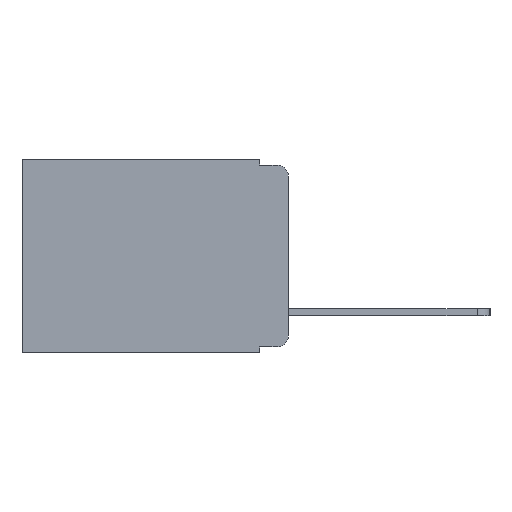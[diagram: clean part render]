
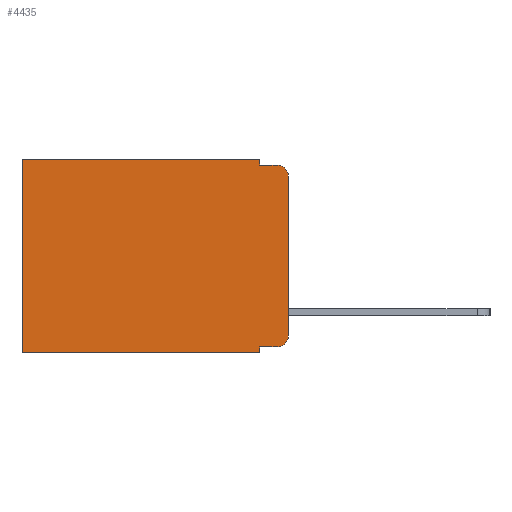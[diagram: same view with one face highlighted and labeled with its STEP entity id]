
A CAD part, left-side view. The second image highlights one B-rep face of the part: STEP entity #4435.
In plain terms, the highlighted planar face has unit normal (-1, 0, 0).
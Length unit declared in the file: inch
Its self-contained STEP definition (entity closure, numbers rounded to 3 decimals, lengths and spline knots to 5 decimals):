
#233 = ORIENTED_EDGE ( 'NONE', *, *, #13296, .F. ) ;
#249 = ORIENTED_EDGE ( 'NONE', *, *, #522, .T. ) ;
#310 = VERTEX_POINT ( 'NONE', #15854 ) ;
#501 = FACE_OUTER_BOUND ( 'NONE', #6008, .T. ) ;
#522 = EDGE_CURVE ( 'NONE', #1548, #3843, #5120, .T. ) ;
#576 = DIRECTION ( 'NONE',  ( 0., 1., 0. ) ) ;
#608 = DIRECTION ( 'NONE',  ( 0., -1., 0. ) ) ;
#623 = CARTESIAN_POINT ( 'NONE',  ( 0.298, 0., 0. ) ) ;
#873 = ORIENTED_EDGE ( 'NONE', *, *, #13072, .T. ) ;
#1028 = ORIENTED_EDGE ( 'NONE', *, *, #13233, .F. ) ;
#1104 = DIRECTION ( 'NONE',  ( 0., 0., -1. ) ) ;
#1265 = CARTESIAN_POINT ( 'NONE',  ( 0.298, 0., 0. ) ) ;
#1548 = VERTEX_POINT ( 'NONE', #4583 ) ;
#1913 = VERTEX_POINT ( 'NONE', #6300 ) ;
#2069 = ORIENTED_EDGE ( 'NONE', *, *, #13324, .T. ) ;
#2408 = VECTOR ( 'NONE', #576, 39.37008 ) ;
#3073 = VERTEX_POINT ( 'NONE', #6090 ) ;
#3367 = ORIENTED_EDGE ( 'NONE', *, *, #11075, .F. ) ;
#3386 = DIRECTION ( 'NONE',  ( 0., 1., 0. ) ) ;
#3620 = VECTOR ( 'NONE', #6808, 39.37008 ) ;
#3739 = CARTESIAN_POINT ( 'NONE',  ( 0.298, 0.051, -0.333 ) ) ;
#3843 = VERTEX_POINT ( 'NONE', #13673 ) ;
#4435 = ADVANCED_FACE ( 'NONE', ( #501 ), #11985, .F. ) ;
#4469 = DIRECTION ( 'NONE',  ( 0., 0., -1. ) ) ;
#4554 = CARTESIAN_POINT ( 'NONE',  ( 0.298, 0.473, -0.343 ) ) ;
#4583 = CARTESIAN_POINT ( 'NONE',  ( 0.298, 0.051, 0. ) ) ;
#4594 = LINE ( 'NONE', #18398, #18764 ) ;
#4664 = DIRECTION ( 'NONE',  ( -1., 0., 0. ) ) ;
#4992 = ORIENTED_EDGE ( 'NONE', *, *, #13290, .T. ) ;
#5120 = LINE ( 'NONE', #623, #2408 ) ;
#5637 = ORIENTED_EDGE ( 'NONE', *, *, #13431, .T. ) ;
#5700 = AXIS2_PLACEMENT_3D ( 'NONE', #18890, #10250, #1104 ) ;
#6008 = EDGE_LOOP ( 'NONE', ( #17667, #873, #18795, #1028, #249, #4992, #3367, #233, #2069, #5637 ) ) ;
#6090 = CARTESIAN_POINT ( 'NONE',  ( 0.298, 0., -0.03 ) ) ;
#6300 = CARTESIAN_POINT ( 'NONE',  ( 0.298, 0.02, -0.01 ) ) ;
#6516 = DIRECTION ( 'NONE',  ( 1., 0., 0. ) ) ;
#6535 = DIRECTION ( 'NONE',  ( 0., 0., -1. ) ) ;
#6622 = CARTESIAN_POINT ( 'NONE',  ( 0.298, 0.051, 0. ) ) ;
#6697 = LINE ( 'NONE', #8375, #14943 ) ;
#6808 = DIRECTION ( 'NONE',  ( 0., 0., -1. ) ) ;
#7389 = CIRCLE ( 'NONE', #5700, 0.02 ) ;
#7583 = VERTEX_POINT ( 'NONE', #4554 ) ;
#7874 = DIRECTION ( 'NONE',  ( 0., -1., 0. ) ) ;
#7884 = AXIS2_PLACEMENT_3D ( 'NONE', #10514, #6516, #6535 ) ;
#8375 = CARTESIAN_POINT ( 'NONE',  ( 0.298, 0.051, -0.333 ) ) ;
#8570 = VERTEX_POINT ( 'NONE', #12175 ) ;
#8960 = CARTESIAN_POINT ( 'NONE',  ( 0.298, 0., -0.313 ) ) ;
#9608 = DIRECTION ( 'NONE',  ( 0., 0., -1. ) ) ;
#9620 = VERTEX_POINT ( 'NONE', #12366 ) ;
#9735 = DIRECTION ( 'NONE',  ( 0., 0., -1. ) ) ;
#9737 = VECTOR ( 'NONE', #4469, 39.37008 ) ;
#10250 = DIRECTION ( 'NONE',  ( -1., 0., 0. ) ) ;
#10514 = CARTESIAN_POINT ( 'NONE',  ( 0.298, 0., 0. ) ) ;
#10768 = CARTESIAN_POINT ( 'NONE',  ( 0.298, 0.051, -0.01 ) ) ;
#11075 = EDGE_CURVE ( 'NONE', #8570, #7583, #19067, .T. ) ;
#11560 = LINE ( 'NONE', #15562, #3620 ) ;
#11610 = VERTEX_POINT ( 'NONE', #8960 ) ;
#11985 = PLANE ( 'NONE',  #7884 ) ;
#12009 = VECTOR ( 'NONE', #9608, 39.37008 ) ;
#12175 = CARTESIAN_POINT ( 'NONE',  ( 0.298, 0.051, -0.343 ) ) ;
#12366 = CARTESIAN_POINT ( 'NONE',  ( 0.298, 0.051, -0.01 ) ) ;
#13004 = EDGE_CURVE ( 'NONE', #3073, #11610, #13596, .T. ) ;
#13072 = EDGE_CURVE ( 'NONE', #3073, #1913, #16098, .T. ) ;
#13150 = EDGE_CURVE ( 'NONE', #9620, #1913, #18117, .T. ) ;
#13233 = EDGE_CURVE ( 'NONE', #1548, #9620, #16319, .T. ) ;
#13290 = EDGE_CURVE ( 'NONE', #3843, #7583, #4594, .T. ) ;
#13296 = EDGE_CURVE ( 'NONE', #15083, #8570, #11560, .T. ) ;
#13319 = AXIS2_PLACEMENT_3D ( 'NONE', #13483, #4664, #14945 ) ;
#13324 = EDGE_CURVE ( 'NONE', #15083, #310, #6697, .T. ) ;
#13431 = EDGE_CURVE ( 'NONE', #310, #11610, #7389, .T. ) ;
#13483 = CARTESIAN_POINT ( 'NONE',  ( 0.298, 0.02, -0.03 ) ) ;
#13596 = LINE ( 'NONE', #1265, #9737 ) ;
#13673 = CARTESIAN_POINT ( 'NONE',  ( 0.298, 0.473, 0. ) ) ;
#14283 = VECTOR ( 'NONE', #7874, 39.37008 ) ;
#14943 = VECTOR ( 'NONE', #608, 39.37008 ) ;
#14945 = DIRECTION ( 'NONE',  ( 0., 0., -1. ) ) ;
#15083 = VERTEX_POINT ( 'NONE', #3739 ) ;
#15246 = VECTOR ( 'NONE', #3386, 39.37008 ) ;
#15562 = CARTESIAN_POINT ( 'NONE',  ( 0.298, 0.051, 0. ) ) ;
#15854 = CARTESIAN_POINT ( 'NONE',  ( 0.298, 0.02, -0.333 ) ) ;
#16098 = CIRCLE ( 'NONE', #13319, 0.02 ) ;
#16319 = LINE ( 'NONE', #6622, #12009 ) ;
#17667 = ORIENTED_EDGE ( 'NONE', *, *, #13004, .F. ) ;
#18056 = CARTESIAN_POINT ( 'NONE',  ( 0.298, 0., -0.343 ) ) ;
#18117 = LINE ( 'NONE', #10768, #14283 ) ;
#18398 = CARTESIAN_POINT ( 'NONE',  ( 0.298, 0.473, 0. ) ) ;
#18764 = VECTOR ( 'NONE', #9735, 39.37008 ) ;
#18795 = ORIENTED_EDGE ( 'NONE', *, *, #13150, .F. ) ;
#18890 = CARTESIAN_POINT ( 'NONE',  ( 0.298, 0.02, -0.313 ) ) ;
#19067 = LINE ( 'NONE', #18056, #15246 ) ;
